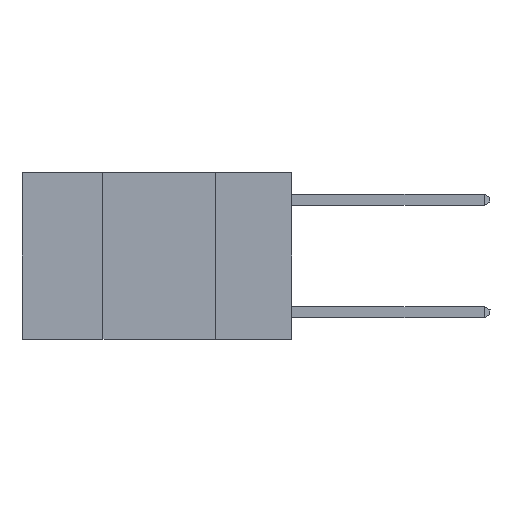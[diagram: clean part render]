
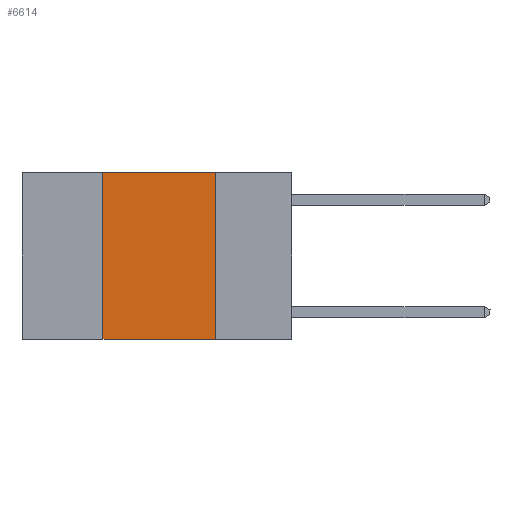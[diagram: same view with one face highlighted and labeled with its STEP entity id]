
A CAD part, left-side view. The second image highlights one B-rep face of the part: STEP entity #6614.
In plain terms, the highlighted planar face has unit normal (-1, 0, 0).
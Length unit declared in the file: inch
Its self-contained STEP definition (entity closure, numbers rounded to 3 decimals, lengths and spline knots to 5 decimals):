
#198 = CARTESIAN_POINT ( 'NONE',  ( 0., 0.17, -0.37 ) ) ;
#301 = DIRECTION ( 'NONE',  ( 0., 0., -1. ) ) ;
#353 = ORIENTED_EDGE ( 'NONE', *, *, #20546, .F. ) ;
#948 = VECTOR ( 'NONE', #13405, 39.37008 ) ;
#3934 = FACE_OUTER_BOUND ( 'NONE', #23851, .T. ) ;
#6614 = ADVANCED_FACE ( 'NONE', ( #3934 ), #25719, .F. ) ;
#7507 = DIRECTION ( 'NONE',  ( 0., 0., 1. ) ) ;
#8604 = VERTEX_POINT ( 'NONE', #198 ) ;
#8612 = EDGE_CURVE ( 'NONE', #26031, #8604, #10636, .T. ) ;
#9661 = AXIS2_PLACEMENT_3D ( 'NONE', #14145, #11926, #28011 ) ;
#9878 = ORIENTED_EDGE ( 'NONE', *, *, #25402, .T. ) ;
#10234 = VECTOR ( 'NONE', #7507, 39.37008 ) ;
#10636 = LINE ( 'NONE', #25499, #28239 ) ;
#11912 = VERTEX_POINT ( 'NONE', #25250 ) ;
#11926 = DIRECTION ( 'NONE',  ( 1., 0., 0. ) ) ;
#12475 = CARTESIAN_POINT ( 'NONE',  ( 0., 0.42, 0. ) ) ;
#12497 = CARTESIAN_POINT ( 'NONE',  ( 0., 0.6, -0.37 ) ) ;
#13405 = DIRECTION ( 'NONE',  ( 0., -1., 0. ) ) ;
#14145 = CARTESIAN_POINT ( 'NONE',  ( 0., 0.6, 0. ) ) ;
#14275 = VECTOR ( 'NONE', #17005, 39.37008 ) ;
#16254 = ORIENTED_EDGE ( 'NONE', *, *, #8612, .F. ) ;
#17005 = DIRECTION ( 'NONE',  ( 0., -1., 0. ) ) ;
#18947 = CARTESIAN_POINT ( 'NONE',  ( 0., 0.42, 0. ) ) ;
#19050 = VERTEX_POINT ( 'NONE', #12475 ) ;
#20546 = EDGE_CURVE ( 'NONE', #19050, #26031, #23943, .T. ) ;
#23619 = CARTESIAN_POINT ( 'NONE',  ( 0., 0.17, 0. ) ) ;
#23851 = EDGE_LOOP ( 'NONE', ( #16254, #353, #26662, #9878 ) ) ;
#23943 = LINE ( 'NONE', #27183, #948 ) ;
#25250 = CARTESIAN_POINT ( 'NONE',  ( 0., 0.42, -0.37 ) ) ;
#25402 = EDGE_CURVE ( 'NONE', #11912, #8604, #26521, .T. ) ;
#25499 = CARTESIAN_POINT ( 'NONE',  ( 0., 0.17, 0. ) ) ;
#25719 = PLANE ( 'NONE',  #9661 ) ;
#26031 = VERTEX_POINT ( 'NONE', #23619 ) ;
#26521 = LINE ( 'NONE', #12497, #14275 ) ;
#26662 = ORIENTED_EDGE ( 'NONE', *, *, #26747, .F. ) ;
#26747 = EDGE_CURVE ( 'NONE', #11912, #19050, #27851, .T. ) ;
#27183 = CARTESIAN_POINT ( 'NONE',  ( 0., 0.6, 0. ) ) ;
#27851 = LINE ( 'NONE', #18947, #10234 ) ;
#28011 = DIRECTION ( 'NONE',  ( 0., 0., -1. ) ) ;
#28239 = VECTOR ( 'NONE', #301, 39.37008 ) ;
